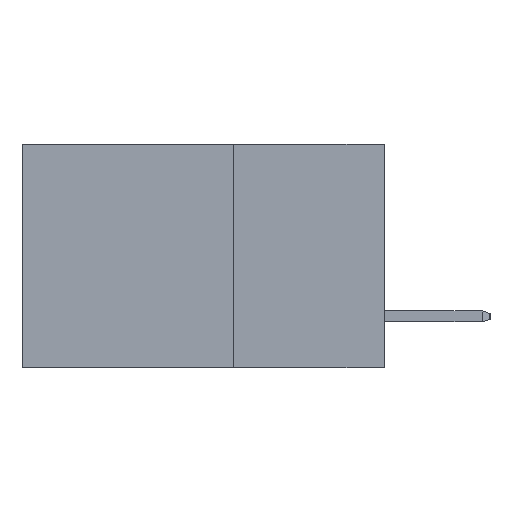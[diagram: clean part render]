
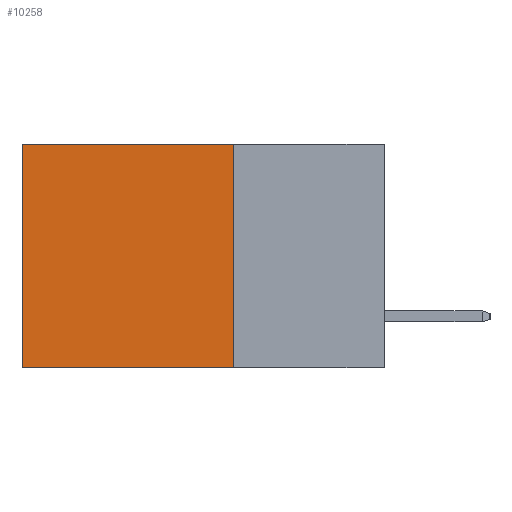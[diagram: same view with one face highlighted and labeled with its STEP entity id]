
A CAD part, left-side view. The second image highlights one B-rep face of the part: STEP entity #10258.
In plain terms, the highlighted planar face has unit normal (-1, 0, 0).
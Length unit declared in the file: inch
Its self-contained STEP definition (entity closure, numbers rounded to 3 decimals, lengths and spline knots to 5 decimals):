
#1066 = VECTOR ( 'NONE', #11440, 39.37008 ) ;
#2776 = DIRECTION ( 'NONE',  ( 0., 0., -1. ) ) ;
#4155 = EDGE_LOOP ( 'NONE', ( #6126, #10987, #5412, #16161 ) ) ;
#4793 = PLANE ( 'NONE',  #13684 ) ;
#5412 = ORIENTED_EDGE ( 'NONE', *, *, #14994, .F. ) ;
#5479 = CARTESIAN_POINT ( 'NONE',  ( 0.298, 0.6, 0. ) ) ;
#6126 = ORIENTED_EDGE ( 'NONE', *, *, #7179, .T. ) ;
#7071 = LINE ( 'NONE', #17753, #17720 ) ;
#7179 = EDGE_CURVE ( 'NONE', #16527, #22531, #22287, .T. ) ;
#7569 = EDGE_CURVE ( 'NONE', #20280, #16527, #7071, .T. ) ;
#8901 = DIRECTION ( 'NONE',  ( 1., 0., 0. ) ) ;
#9142 = FACE_OUTER_BOUND ( 'NONE', #4155, .T. ) ;
#10258 = ADVANCED_FACE ( 'NONE', ( #9142 ), #4793, .F. ) ;
#10987 = ORIENTED_EDGE ( 'NONE', *, *, #21952, .F. ) ;
#11440 = DIRECTION ( 'NONE',  ( 0., 0., -1. ) ) ;
#12388 = LINE ( 'NONE', #24167, #17682 ) ;
#12447 = DIRECTION ( 'NONE',  ( 0., 1., 0. ) ) ;
#12900 = CARTESIAN_POINT ( 'NONE',  ( 0.298, 0.25, 0. ) ) ;
#13684 = AXIS2_PLACEMENT_3D ( 'NONE', #18842, #8901, #22717 ) ;
#14994 = EDGE_CURVE ( 'NONE', #20280, #20098, #24527, .T. ) ;
#16161 = ORIENTED_EDGE ( 'NONE', *, *, #7569, .T. ) ;
#16360 = CARTESIAN_POINT ( 'NONE',  ( 0.298, 0.6, -0.37 ) ) ;
#16527 = VERTEX_POINT ( 'NONE', #25556 ) ;
#17678 = DIRECTION ( 'NONE',  ( 0., 1., 0. ) ) ;
#17682 = VECTOR ( 'NONE', #12447, 39.37008 ) ;
#17720 = VECTOR ( 'NONE', #17678, 39.37008 ) ;
#17753 = CARTESIAN_POINT ( 'NONE',  ( 0.298, 0.25, 0. ) ) ;
#18507 = CARTESIAN_POINT ( 'NONE',  ( 0.298, 0.25, -0.37 ) ) ;
#18842 = CARTESIAN_POINT ( 'NONE',  ( 0.298, 0.25, 0. ) ) ;
#20098 = VERTEX_POINT ( 'NONE', #18507 ) ;
#20280 = VERTEX_POINT ( 'NONE', #24841 ) ;
#21952 = EDGE_CURVE ( 'NONE', #20098, #22531, #12388, .T. ) ;
#22287 = LINE ( 'NONE', #5479, #1066 ) ;
#22531 = VERTEX_POINT ( 'NONE', #16360 ) ;
#22717 = DIRECTION ( 'NONE',  ( 0., 0., -1. ) ) ;
#23901 = VECTOR ( 'NONE', #2776, 39.37008 ) ;
#24167 = CARTESIAN_POINT ( 'NONE',  ( 0.298, 0.25, -0.37 ) ) ;
#24527 = LINE ( 'NONE', #12900, #23901 ) ;
#24841 = CARTESIAN_POINT ( 'NONE',  ( 0.298, 0.25, 0. ) ) ;
#25556 = CARTESIAN_POINT ( 'NONE',  ( 0.298, 0.6, 0. ) ) ;
